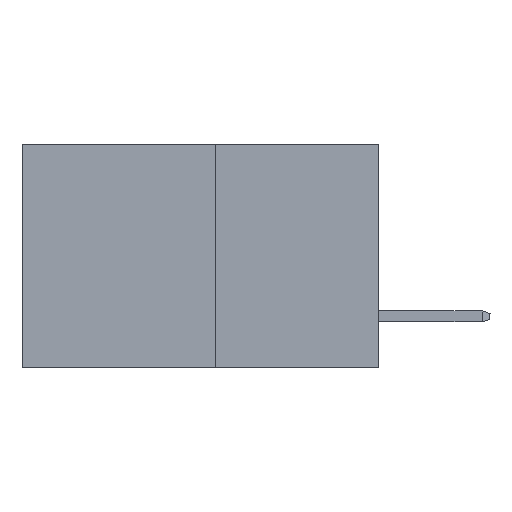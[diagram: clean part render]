
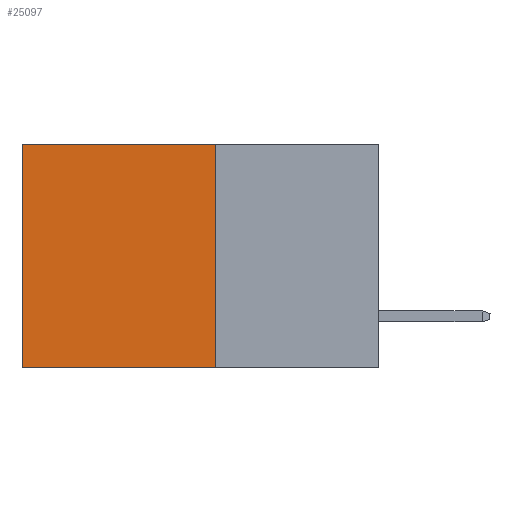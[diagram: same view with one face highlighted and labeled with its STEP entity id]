
A CAD part, left-side view. The second image highlights one B-rep face of the part: STEP entity #25097.
In plain terms, the highlighted planar face has unit normal (-1, 0, 0).
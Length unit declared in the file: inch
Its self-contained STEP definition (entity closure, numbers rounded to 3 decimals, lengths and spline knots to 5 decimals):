
#800 = DIRECTION ( 'NONE',  ( 1., 0., 0. ) ) ;
#877 = ORIENTED_EDGE ( 'NONE', *, *, #6569, .F. ) ;
#2246 = ORIENTED_EDGE ( 'NONE', *, *, #28420, .T. ) ;
#2467 = CARTESIAN_POINT ( 'NONE',  ( 0.277, 0.59, -0.37 ) ) ;
#4977 = ORIENTED_EDGE ( 'NONE', *, *, #5322, .T. ) ;
#5256 = CARTESIAN_POINT ( 'NONE',  ( 0.277, 0.27, -0.37 ) ) ;
#5322 = EDGE_CURVE ( 'NONE', #27489, #8198, #18323, .T. ) ;
#5393 = VECTOR ( 'NONE', #26281, 39.37008 ) ;
#6569 = EDGE_CURVE ( 'NONE', #27489, #19676, #15063, .T. ) ;
#6930 = AXIS2_PLACEMENT_3D ( 'NONE', #12202, #800, #16905 ) ;
#7669 = PLANE ( 'NONE',  #6930 ) ;
#8198 = VERTEX_POINT ( 'NONE', #22697 ) ;
#8999 = LINE ( 'NONE', #18120, #14407 ) ;
#12112 = CARTESIAN_POINT ( 'NONE',  ( 0.277, 0.27, -0.37 ) ) ;
#12202 = CARTESIAN_POINT ( 'NONE',  ( 0.277, 0.27, -0.37 ) ) ;
#12595 = CARTESIAN_POINT ( 'NONE',  ( 0.277, 0.27, 0. ) ) ;
#14407 = VECTOR ( 'NONE', #20312, 39.37008 ) ;
#14533 = DIRECTION ( 'NONE',  ( 0., 1., 0. ) ) ;
#15063 = LINE ( 'NONE', #24101, #20301 ) ;
#16905 = DIRECTION ( 'NONE',  ( 0., 0., -1. ) ) ;
#18120 = CARTESIAN_POINT ( 'NONE',  ( 0.277, 0.59, -0.37 ) ) ;
#18209 = FACE_OUTER_BOUND ( 'NONE', #24787, .T. ) ;
#18323 = LINE ( 'NONE', #26518, #5393 ) ;
#18898 = VERTEX_POINT ( 'NONE', #2467 ) ;
#19360 = LINE ( 'NONE', #5256, #24420 ) ;
#19676 = VERTEX_POINT ( 'NONE', #12112 ) ;
#19773 = DIRECTION ( 'NONE',  ( 0., 0., -1. ) ) ;
#19812 = ORIENTED_EDGE ( 'NONE', *, *, #23210, .F. ) ;
#20301 = VECTOR ( 'NONE', #19773, 39.37008 ) ;
#20312 = DIRECTION ( 'NONE',  ( 0., 0., -1. ) ) ;
#22697 = CARTESIAN_POINT ( 'NONE',  ( 0.277, 0.59, 0. ) ) ;
#23210 = EDGE_CURVE ( 'NONE', #19676, #18898, #19360, .T. ) ;
#24101 = CARTESIAN_POINT ( 'NONE',  ( 0.277, 0.27, -0.37 ) ) ;
#24420 = VECTOR ( 'NONE', #14533, 39.37008 ) ;
#24787 = EDGE_LOOP ( 'NONE', ( #2246, #19812, #877, #4977 ) ) ;
#25097 = ADVANCED_FACE ( 'NONE', ( #18209 ), #7669, .F. ) ;
#26281 = DIRECTION ( 'NONE',  ( 0., 1., 0. ) ) ;
#26518 = CARTESIAN_POINT ( 'NONE',  ( 0.277, 0.27, 0. ) ) ;
#27489 = VERTEX_POINT ( 'NONE', #12595 ) ;
#28420 = EDGE_CURVE ( 'NONE', #8198, #18898, #8999, .T. ) ;
